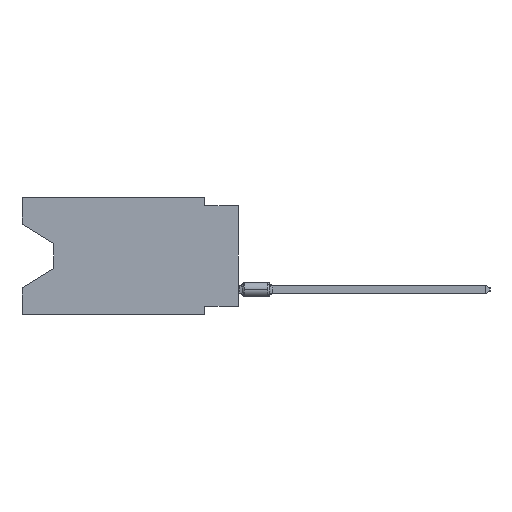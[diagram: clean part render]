
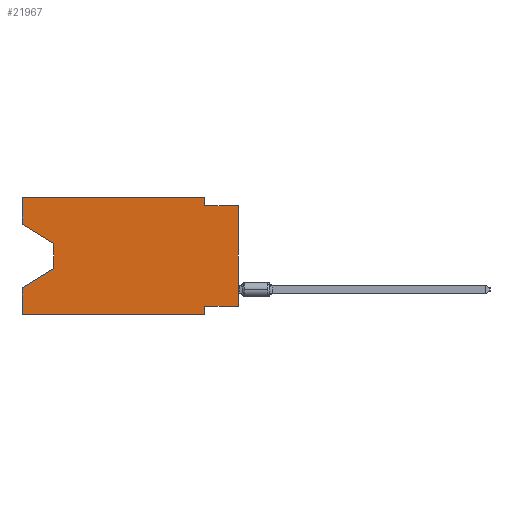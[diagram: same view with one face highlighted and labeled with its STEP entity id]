
A CAD part, left-side view. The second image highlights one B-rep face of the part: STEP entity #21967.
In plain terms, the highlighted planar face has unit normal (-1, 0, 0).
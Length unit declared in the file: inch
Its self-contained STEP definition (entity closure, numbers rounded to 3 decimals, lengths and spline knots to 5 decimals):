
#214 = CARTESIAN_POINT ( 'NONE',  ( 0., 0.1, -0.35 ) ) ;
#404 = LINE ( 'NONE', #15163, #16486 ) ;
#767 = CARTESIAN_POINT ( 'NONE',  ( 0., 0.1, -0.325 ) ) ;
#769 = VERTEX_POINT ( 'NONE', #767 ) ;
#1531 = EDGE_CURVE ( 'NONE', #30725, #25285, #31629, .T. ) ;
#2144 = EDGE_CURVE ( 'NONE', #9318, #34965, #11212, .T. ) ;
#2183 = CARTESIAN_POINT ( 'NONE',  ( 0., 0.645, -0.26975 ) ) ;
#2862 = VECTOR ( 'NONE', #30244, 39.37008 ) ;
#2995 = LINE ( 'NONE', #8737, #17818 ) ;
#3041 = ORIENTED_EDGE ( 'NONE', *, *, #28634, .F. ) ;
#3083 = EDGE_LOOP ( 'NONE', ( #22366, #18190, #10828, #38383, #4744, #37766, #3041, #36357, #10572, #28128, #37258, #18033 ) ) ;
#3487 = DIRECTION ( 'NONE',  ( 0., 0., -1. ) ) ;
#3920 = DIRECTION ( 'NONE',  ( 0., 0., 1. ) ) ;
#4092 = LINE ( 'NONE', #16606, #17941 ) ;
#4258 = CARTESIAN_POINT ( 'NONE',  ( 0., 0.645, -0.08025 ) ) ;
#4285 = VECTOR ( 'NONE', #13893, 39.37008 ) ;
#4744 = ORIENTED_EDGE ( 'NONE', *, *, #30711, .T. ) ;
#6721 = EDGE_CURVE ( 'NONE', #34965, #22217, #20806, .T. ) ;
#7035 = LINE ( 'NONE', #19530, #15511 ) ;
#7662 = CARTESIAN_POINT ( 'NONE',  ( 0., 0.645, 0. ) ) ;
#8737 = CARTESIAN_POINT ( 'NONE',  ( 0., 0., -0.325 ) ) ;
#9318 = VERTEX_POINT ( 'NONE', #13235 ) ;
#9780 = VECTOR ( 'NONE', #39257, 39.37008 ) ;
#10001 = DIRECTION ( 'NONE',  ( 1., 0., 0. ) ) ;
#10276 = CARTESIAN_POINT ( 'NONE',  ( 0., 0.1, 0. ) ) ;
#10572 = ORIENTED_EDGE ( 'NONE', *, *, #26708, .F. ) ;
#10828 = ORIENTED_EDGE ( 'NONE', *, *, #12973, .T. ) ;
#11061 = CARTESIAN_POINT ( 'NONE',  ( 0., 0.645, -0.35 ) ) ;
#11212 = LINE ( 'NONE', #4258, #22608 ) ;
#11599 = DIRECTION ( 'NONE',  ( 0., -1., 0. ) ) ;
#12791 = EDGE_CURVE ( 'NONE', #31961, #22156, #14289, .T. ) ;
#12973 = EDGE_CURVE ( 'NONE', #22217, #22156, #25135, .T. ) ;
#13235 = CARTESIAN_POINT ( 'NONE',  ( 0., 0.645, -0.08025 ) ) ;
#13893 = DIRECTION ( 'NONE',  ( 0., 0., 1. ) ) ;
#14289 = LINE ( 'NONE', #17383, #4285 ) ;
#14619 = CARTESIAN_POINT ( 'NONE',  ( 0., 0.55, -0.138 ) ) ;
#15110 = AXIS2_PLACEMENT_3D ( 'NONE', #28903, #10001, #31788 ) ;
#15126 = VECTOR ( 'NONE', #11599, 39.37008 ) ;
#15163 = CARTESIAN_POINT ( 'NONE',  ( 0., 0., -0.025 ) ) ;
#15415 = VERTEX_POINT ( 'NONE', #22316 ) ;
#15487 = LINE ( 'NONE', #27826, #15126 ) ;
#15511 = VECTOR ( 'NONE', #3920, 39.37008 ) ;
#16471 = DIRECTION ( 'NONE',  ( 0., 0.855, -0.519 ) ) ;
#16486 = VECTOR ( 'NONE', #34088, 39.37008 ) ;
#16606 = CARTESIAN_POINT ( 'NONE',  ( 0., 0.645, -0.35 ) ) ;
#16878 = LINE ( 'NONE', #7662, #9780 ) ;
#17383 = CARTESIAN_POINT ( 'NONE',  ( 0., 0.645, 0. ) ) ;
#17634 = EDGE_CURVE ( 'NONE', #28924, #28376, #7035, .T. ) ;
#17818 = VECTOR ( 'NONE', #22101, 39.37008 ) ;
#17941 = VECTOR ( 'NONE', #28743, 39.37008 ) ;
#18033 = ORIENTED_EDGE ( 'NONE', *, *, #24211, .F. ) ;
#18190 = ORIENTED_EDGE ( 'NONE', *, *, #6721, .T. ) ;
#18535 = CARTESIAN_POINT ( 'NONE',  ( 0., 0.1, -0.35 ) ) ;
#18746 = LINE ( 'NONE', #18535, #37118 ) ;
#18946 = CARTESIAN_POINT ( 'NONE',  ( 0., 0.1, -0.025 ) ) ;
#19530 = CARTESIAN_POINT ( 'NONE',  ( 0., 0., 0. ) ) ;
#20806 = LINE ( 'NONE', #14619, #2862 ) ;
#21291 = CARTESIAN_POINT ( 'NONE',  ( 0., 0.55, -0.212 ) ) ;
#21835 = VECTOR ( 'NONE', #16471, 39.37008 ) ;
#21967 = ADVANCED_FACE ( 'NONE', ( #31581 ), #22337, .F. ) ;
#22101 = DIRECTION ( 'NONE',  ( 0., 1., 0. ) ) ;
#22156 = VERTEX_POINT ( 'NONE', #2183 ) ;
#22217 = VERTEX_POINT ( 'NONE', #21291 ) ;
#22316 = CARTESIAN_POINT ( 'NONE',  ( 0., 0.645, 0. ) ) ;
#22337 = PLANE ( 'NONE',  #15110 ) ;
#22366 = ORIENTED_EDGE ( 'NONE', *, *, #2144, .T. ) ;
#22608 = VECTOR ( 'NONE', #36065, 39.37008 ) ;
#24129 = VECTOR ( 'NONE', #3487, 39.37008 ) ;
#24211 = EDGE_CURVE ( 'NONE', #9318, #15415, #16878, .T. ) ;
#25135 = LINE ( 'NONE', #37668, #21835 ) ;
#25285 = VERTEX_POINT ( 'NONE', #18946 ) ;
#26000 = CARTESIAN_POINT ( 'NONE',  ( 0., 0.55, -0.138 ) ) ;
#26081 = CARTESIAN_POINT ( 'NONE',  ( 0., 0.1, 0. ) ) ;
#26199 = EDGE_CURVE ( 'NONE', #15415, #30725, #15487, .T. ) ;
#26708 = EDGE_CURVE ( 'NONE', #25285, #28376, #404, .T. ) ;
#27826 = CARTESIAN_POINT ( 'NONE',  ( 0., 0.645, 0. ) ) ;
#28128 = ORIENTED_EDGE ( 'NONE', *, *, #1531, .F. ) ;
#28376 = VERTEX_POINT ( 'NONE', #35879 ) ;
#28634 = EDGE_CURVE ( 'NONE', #28924, #769, #2995, .T. ) ;
#28743 = DIRECTION ( 'NONE',  ( 0., -1., 0. ) ) ;
#28903 = CARTESIAN_POINT ( 'NONE',  ( 0., 0.645, 0. ) ) ;
#28924 = VERTEX_POINT ( 'NONE', #40116 ) ;
#29391 = VERTEX_POINT ( 'NONE', #214 ) ;
#30244 = DIRECTION ( 'NONE',  ( 0., 0., -1. ) ) ;
#30711 = EDGE_CURVE ( 'NONE', #31961, #29391, #4092, .T. ) ;
#30725 = VERTEX_POINT ( 'NONE', #26081 ) ;
#31301 = DIRECTION ( 'NONE',  ( 0., 0., -1. ) ) ;
#31581 = FACE_OUTER_BOUND ( 'NONE', #3083, .T. ) ;
#31629 = LINE ( 'NONE', #10276, #24129 ) ;
#31788 = DIRECTION ( 'NONE',  ( 0., 0., -1. ) ) ;
#31961 = VERTEX_POINT ( 'NONE', #11061 ) ;
#32925 = EDGE_CURVE ( 'NONE', #769, #29391, #18746, .T. ) ;
#34088 = DIRECTION ( 'NONE',  ( 0., -1., 0. ) ) ;
#34965 = VERTEX_POINT ( 'NONE', #26000 ) ;
#35879 = CARTESIAN_POINT ( 'NONE',  ( 0., 0., -0.025 ) ) ;
#36065 = DIRECTION ( 'NONE',  ( 0., -0.855, -0.519 ) ) ;
#36357 = ORIENTED_EDGE ( 'NONE', *, *, #17634, .T. ) ;
#37118 = VECTOR ( 'NONE', #31301, 39.37008 ) ;
#37258 = ORIENTED_EDGE ( 'NONE', *, *, #26199, .F. ) ;
#37668 = CARTESIAN_POINT ( 'NONE',  ( 0., 0.55, -0.212 ) ) ;
#37766 = ORIENTED_EDGE ( 'NONE', *, *, #32925, .F. ) ;
#38383 = ORIENTED_EDGE ( 'NONE', *, *, #12791, .F. ) ;
#39257 = DIRECTION ( 'NONE',  ( 0., 0., 1. ) ) ;
#40116 = CARTESIAN_POINT ( 'NONE',  ( 0., 0., -0.325 ) ) ;
